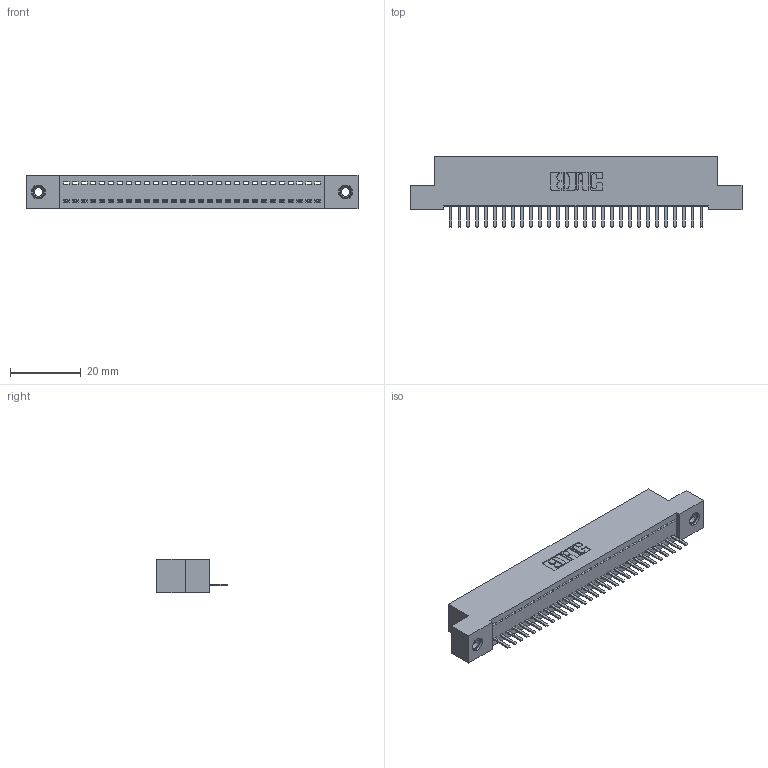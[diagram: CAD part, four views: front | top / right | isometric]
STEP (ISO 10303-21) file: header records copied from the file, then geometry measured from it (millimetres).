
FILE_DESCRIPTION (( 'STEP AP203' ), '1' );
FILE_NAME ('342-029-520-107.STEP', '2019-10-02T03:37:18', ( '' ), ( '' ), 'SwSTEP 2.0', 'SolidWorks 2016', '' );
FILE_SCHEMA (( 'CONFIG_CONTROL_DESIGN' ));
Length unit declared in the file: inch
Products named in the file (4): 345-292-001_345-293-120; 345-250-001_345-250-005-103; 342-029-520-107; 342 Part_TI
Assembly tree (32 placements, depth 2):
  342-029-520-107
    342 Part_TI
    345-292-001_345-293-120  x29
    345-250-001_345-250-005-103  x2
Bounding box: 93.98 x 20.02 x 9.4 mm (x, y, z)
Volume: 8096.2 mm3; surface area: 11411.6 mm2
Topology: 32 solids, 32 shells, 1968 faces, 5771 edges, 3762 vertices
Faces by surface type: plane 1374, cylinder 578, cone 12, torus 4
Entity records: 20578 total; most frequent: CARTESIAN_POINT 3544, ORIENTED_EDGE 3490, DIRECTION 3037, EDGE_CURVE 1745, LINE 1593, VECTOR 1593, VERTEX_POINT 1156, AXIS2_PLACEMENT_3D 722
